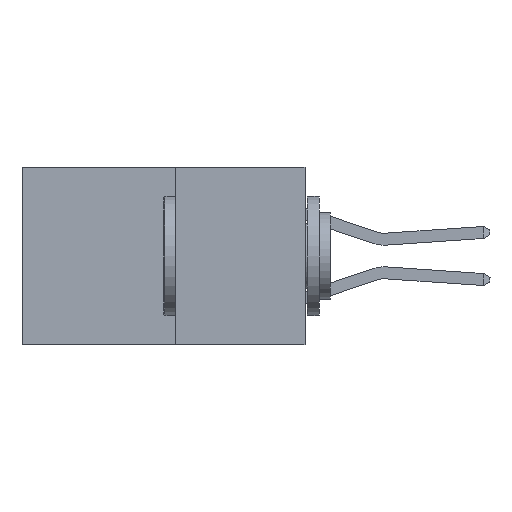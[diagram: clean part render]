
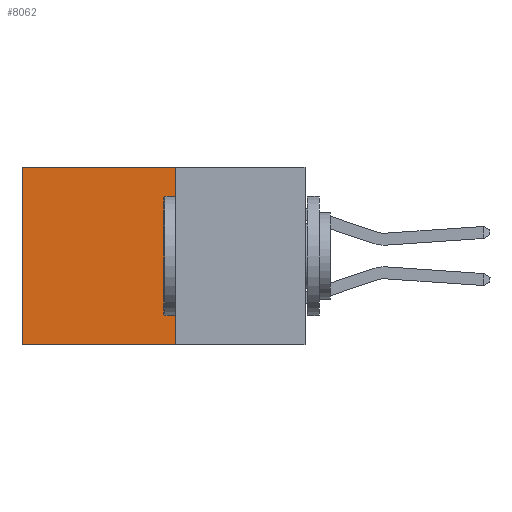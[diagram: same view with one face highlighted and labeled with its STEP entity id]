
A CAD part, left-side view. The second image highlights one B-rep face of the part: STEP entity #8062.
In plain terms, the highlighted planar face has unit normal (-1, 0, 0).
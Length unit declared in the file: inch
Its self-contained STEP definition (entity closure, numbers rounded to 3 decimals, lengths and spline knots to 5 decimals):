
#1164 = VECTOR ( 'NONE', #21370, 39.37008 ) ;
#1309 = DIRECTION ( 'NONE',  ( 0., 0., -1. ) ) ;
#1417 = CARTESIAN_POINT ( 'NONE',  ( 0.277, 0.59, -0.37 ) ) ;
#2471 = AXIS2_PLACEMENT_3D ( 'NONE', #20045, #22632, #7264 ) ;
#2792 = CARTESIAN_POINT ( 'NONE',  ( 0.277, 0.59, -0.37 ) ) ;
#4661 = PLANE ( 'NONE',  #2471 ) ;
#5599 = LINE ( 'NONE', #1417, #11689 ) ;
#5973 = EDGE_CURVE ( 'NONE', #23819, #12872, #5599, .T. ) ;
#6536 = VERTEX_POINT ( 'NONE', #21229 ) ;
#6947 = EDGE_LOOP ( 'NONE', ( #21538, #12333, #19262, #30435 ) ) ;
#7118 = CARTESIAN_POINT ( 'NONE',  ( 0.277, 0.27, 0. ) ) ;
#7264 = DIRECTION ( 'NONE',  ( 0., 0., -1. ) ) ;
#8062 = ADVANCED_FACE ( 'NONE', ( #31835 ), #4661, .F. ) ;
#8611 = VERTEX_POINT ( 'NONE', #7118 ) ;
#10495 = EDGE_CURVE ( 'NONE', #8611, #23819, #21675, .T. ) ;
#11689 = VECTOR ( 'NONE', #1309, 39.37008 ) ;
#12333 = ORIENTED_EDGE ( 'NONE', *, *, #15339, .F. ) ;
#12872 = VERTEX_POINT ( 'NONE', #2792 ) ;
#13308 = DIRECTION ( 'NONE',  ( 0., 1., 0. ) ) ;
#14957 = LINE ( 'NONE', #25210, #27558 ) ;
#15076 = LINE ( 'NONE', #25890, #21071 ) ;
#15339 = EDGE_CURVE ( 'NONE', #6536, #12872, #15076, .T. ) ;
#15398 = CARTESIAN_POINT ( 'NONE',  ( 0.277, 0.59, 0. ) ) ;
#16575 = EDGE_CURVE ( 'NONE', #8611, #6536, #14957, .T. ) ;
#18774 = CARTESIAN_POINT ( 'NONE',  ( 0.277, 0.27, 0. ) ) ;
#19262 = ORIENTED_EDGE ( 'NONE', *, *, #16575, .F. ) ;
#20045 = CARTESIAN_POINT ( 'NONE',  ( 0.277, 0.27, -0.37 ) ) ;
#20276 = DIRECTION ( 'NONE',  ( 0., 0., -1. ) ) ;
#21071 = VECTOR ( 'NONE', #13308, 39.37008 ) ;
#21229 = CARTESIAN_POINT ( 'NONE',  ( 0.277, 0.27, -0.37 ) ) ;
#21370 = DIRECTION ( 'NONE',  ( 0., 1., 0. ) ) ;
#21538 = ORIENTED_EDGE ( 'NONE', *, *, #5973, .T. ) ;
#21675 = LINE ( 'NONE', #18774, #1164 ) ;
#22632 = DIRECTION ( 'NONE',  ( 1., 0., 0. ) ) ;
#23819 = VERTEX_POINT ( 'NONE', #15398 ) ;
#25210 = CARTESIAN_POINT ( 'NONE',  ( 0.277, 0.27, -0.37 ) ) ;
#25890 = CARTESIAN_POINT ( 'NONE',  ( 0.277, 0.27, -0.37 ) ) ;
#27558 = VECTOR ( 'NONE', #20276, 39.37008 ) ;
#30435 = ORIENTED_EDGE ( 'NONE', *, *, #10495, .T. ) ;
#31835 = FACE_OUTER_BOUND ( 'NONE', #6947, .T. ) ;
